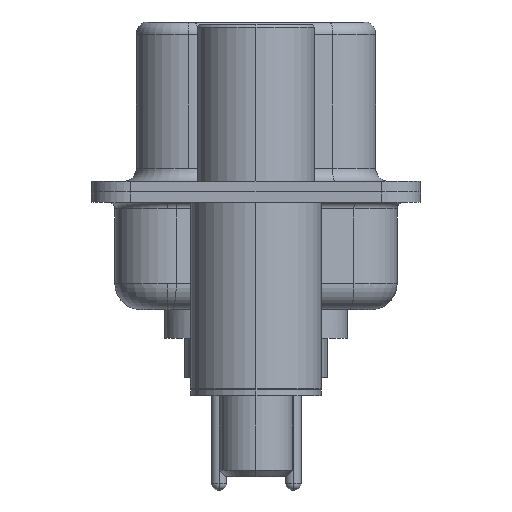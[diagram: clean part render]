
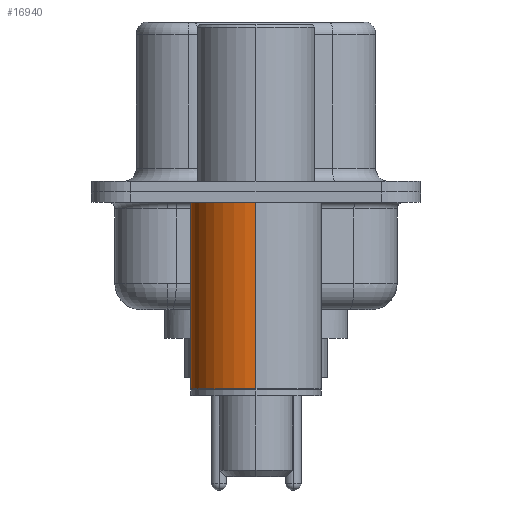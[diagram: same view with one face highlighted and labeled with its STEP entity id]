
A CAD part, left-side view. The second image highlights one B-rep face of the part: STEP entity #16940.
In plain terms, the highlighted cylindrical face has radius 2.5 mm (diameter 5 mm), a partial arc.
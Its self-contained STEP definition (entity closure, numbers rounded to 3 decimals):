
#416 = CARTESIAN_POINT ( 'NONE',  ( 0., 0., 0.581 ) ) ;
#465 = ORIENTED_EDGE ( 'NONE', *, *, #11193, .F. ) ;
#738 = ORIENTED_EDGE ( 'NONE', *, *, #11332, .T. ) ;
#1284 = DIRECTION ( 'NONE',  ( 1., 0., 0. ) ) ;
#1338 = DIRECTION ( 'NONE',  ( 0., 0., 1. ) ) ;
#1458 = DIRECTION ( 'NONE',  ( 1., 0., 0. ) ) ;
#1475 = CARTESIAN_POINT ( 'NONE',  ( 0., 0., -0.4 ) ) ;
#1525 = DIRECTION ( 'NONE',  ( 0., 0., 1. ) ) ;
#1526 = DIRECTION ( 'NONE',  ( 0., 0., 1. ) ) ;
#1584 = CARTESIAN_POINT ( 'NONE',  ( 0., 0., -7.525 ) ) ;
#1840 = CARTESIAN_POINT ( 'NONE',  ( 2.5, 0., 0.581 ) ) ;
#3160 = EDGE_LOOP ( 'NONE', ( #738, #10022, #10573, #465 ) ) ;
#3845 = CARTESIAN_POINT ( 'NONE',  ( -2.5, 0., 0.581 ) ) ;
#4155 = DIRECTION ( 'NONE',  ( 0., 0., 1. ) ) ;
#4950 = VERTEX_POINT ( 'NONE', #18174 ) ;
#7229 = CYLINDRICAL_SURFACE ( 'NONE', #12512, 2.5 ) ;
#7690 = FACE_OUTER_BOUND ( 'NONE', #3160, .T. ) ;
#7885 = DIRECTION ( 'NONE',  ( 1., 0., 0. ) ) ;
#8608 = AXIS2_PLACEMENT_3D ( 'NONE', #1584, #1525, #1458 ) ;
#8816 = VERTEX_POINT ( 'NONE', #17982 ) ;
#9054 = VECTOR ( 'NONE', #1526, 1000. ) ;
#9247 = AXIS2_PLACEMENT_3D ( 'NONE', #1475, #1338, #1284 ) ;
#9504 = VECTOR ( 'NONE', #4155, 1000. ) ;
#9983 = LINE ( 'NONE', #3845, #9504 ) ;
#10022 = ORIENTED_EDGE ( 'NONE', *, *, #11169, .T. ) ;
#10195 = CIRCLE ( 'NONE', #8608, 2.5 ) ;
#10573 = ORIENTED_EDGE ( 'NONE', *, *, #11190, .F. ) ;
#10824 = DIRECTION ( 'NONE',  ( 0., 0., 1. ) ) ;
#11169 = EDGE_CURVE ( 'NONE', #8816, #18153, #9983, .T. ) ;
#11190 = EDGE_CURVE ( 'NONE', #4950, #18153, #16826, .T. ) ;
#11193 = EDGE_CURVE ( 'NONE', #15368, #4950, #13407, .T. ) ;
#11332 = EDGE_CURVE ( 'NONE', #15368, #8816, #10195, .T. ) ;
#12512 = AXIS2_PLACEMENT_3D ( 'NONE', #416, #10824, #7885 ) ;
#13291 = CARTESIAN_POINT ( 'NONE',  ( 2.5, 0., -7.525 ) ) ;
#13407 = LINE ( 'NONE', #1840, #9054 ) ;
#15368 = VERTEX_POINT ( 'NONE', #13291 ) ;
#16826 = CIRCLE ( 'NONE', #9247, 2.5 ) ;
#16940 = ADVANCED_FACE ( 'NONE', ( #7690 ), #7229, .T. ) ;
#17982 = CARTESIAN_POINT ( 'NONE',  ( -2.5, 0., -7.525 ) ) ;
#18153 = VERTEX_POINT ( 'NONE', #19081 ) ;
#18174 = CARTESIAN_POINT ( 'NONE',  ( 2.5, 0., -0.4 ) ) ;
#19081 = CARTESIAN_POINT ( 'NONE',  ( -2.5, 0., -0.4 ) ) ;
